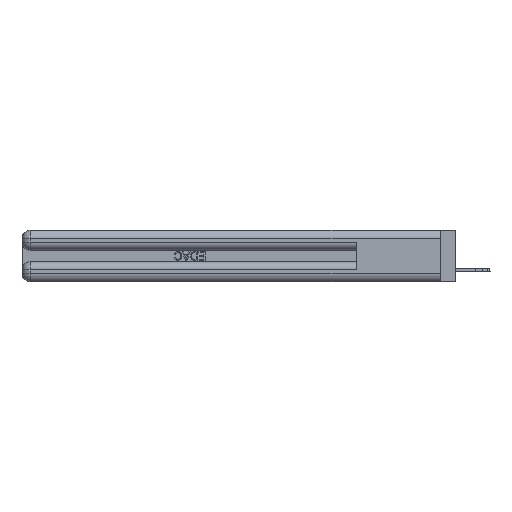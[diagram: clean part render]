
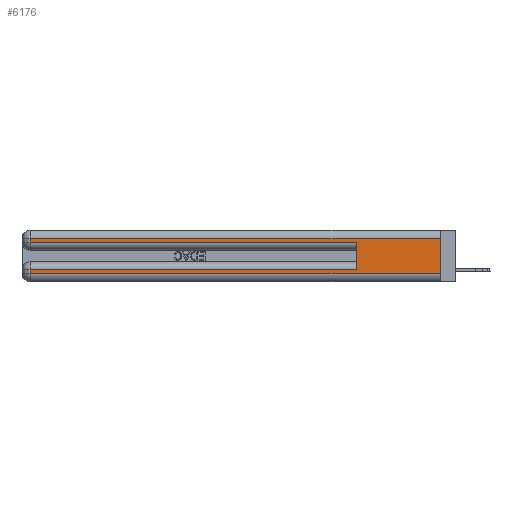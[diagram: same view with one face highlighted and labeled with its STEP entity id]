
A CAD part, left-side view. The second image highlights one B-rep face of the part: STEP entity #6176.
In plain terms, the highlighted planar face has unit normal (-1, 0, 0).
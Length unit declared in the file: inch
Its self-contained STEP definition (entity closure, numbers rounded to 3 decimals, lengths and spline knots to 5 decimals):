
#137 = VECTOR ( 'NONE', #31216, 39.37008 ) ;
#345 = LINE ( 'NONE', #1351, #2214 ) ;
#438 = CARTESIAN_POINT ( 'NONE',  ( 0., 2.94, 0.31 ) ) ;
#1036 = VERTEX_POINT ( 'NONE', #12474 ) ;
#1351 = CARTESIAN_POINT ( 'NONE',  ( 0., 0., 0.06 ) ) ;
#2214 = VECTOR ( 'NONE', #32761, 39.37008 ) ;
#3467 = EDGE_CURVE ( 'NONE', #27188, #27209, #14684, .T. ) ;
#3715 = CARTESIAN_POINT ( 'NONE',  ( 0., 0., 0.085 ) ) ;
#4035 = CARTESIAN_POINT ( 'NONE',  ( 0., 2.94, 0.37 ) ) ;
#4334 = VECTOR ( 'NONE', #23297, 39.37008 ) ;
#4634 = VERTEX_POINT ( 'NONE', #15870 ) ;
#5764 = VECTOR ( 'NONE', #19563, 39.37008 ) ;
#5953 = EDGE_CURVE ( 'NONE', #27188, #14631, #26612, .T. ) ;
#6176 = ADVANCED_FACE ( 'NONE', ( #19824 ), #19379, .F. ) ;
#6967 = CARTESIAN_POINT ( 'NONE',  ( 0., 0., 0.31 ) ) ;
#7120 = VECTOR ( 'NONE', #9620, 39.37008 ) ;
#7391 = ORIENTED_EDGE ( 'NONE', *, *, #26085, .T. ) ;
#7917 = CARTESIAN_POINT ( 'NONE',  ( 0., 0., 0.37 ) ) ;
#8998 = CARTESIAN_POINT ( 'NONE',  ( 0., 0., 0.06 ) ) ;
#9620 = DIRECTION ( 'NONE',  ( 0., 0., -1. ) ) ;
#10275 = LINE ( 'NONE', #4035, #7120 ) ;
#12474 = CARTESIAN_POINT ( 'NONE',  ( 0., 0.6, 0.285 ) ) ;
#12992 = LINE ( 'NONE', #3715, #25179 ) ;
#13042 = EDGE_LOOP ( 'NONE', ( #15852, #16798, #23160, #28432, #29579, #7391, #15346, #23369 ) ) ;
#14120 = AXIS2_PLACEMENT_3D ( 'NONE', #22549, #36945, #28385 ) ;
#14631 = VERTEX_POINT ( 'NONE', #438 ) ;
#14677 = EDGE_CURVE ( 'NONE', #34842, #27209, #345, .T. ) ;
#14684 = LINE ( 'NONE', #7917, #4334 ) ;
#15006 = EDGE_CURVE ( 'NONE', #4634, #1036, #29665, .T. ) ;
#15346 = ORIENTED_EDGE ( 'NONE', *, *, #29931, .T. ) ;
#15852 = ORIENTED_EDGE ( 'NONE', *, *, #3467, .F. ) ;
#15870 = CARTESIAN_POINT ( 'NONE',  ( 0., 2.94, 0.285 ) ) ;
#16798 = ORIENTED_EDGE ( 'NONE', *, *, #5953, .T. ) ;
#17837 = CARTESIAN_POINT ( 'NONE',  ( 0., 2.94, 0.06 ) ) ;
#19379 = PLANE ( 'NONE',  #14120 ) ;
#19454 = EDGE_CURVE ( 'NONE', #14631, #4634, #10275, .T. ) ;
#19563 = DIRECTION ( 'NONE',  ( 0., -1., 0. ) ) ;
#19824 = FACE_OUTER_BOUND ( 'NONE', #13042, .T. ) ;
#21332 = DIRECTION ( 'NONE',  ( 0., 1., 0. ) ) ;
#22549 = CARTESIAN_POINT ( 'NONE',  ( 0., 0., 0.37 ) ) ;
#23160 = ORIENTED_EDGE ( 'NONE', *, *, #19454, .T. ) ;
#23297 = DIRECTION ( 'NONE',  ( 0., 0., -1. ) ) ;
#23369 = ORIENTED_EDGE ( 'NONE', *, *, #14677, .T. ) ;
#25179 = VECTOR ( 'NONE', #21332, 39.37008 ) ;
#25844 = LINE ( 'NONE', #34040, #137 ) ;
#26085 = EDGE_CURVE ( 'NONE', #35546, #35558, #12992, .T. ) ;
#26132 = EDGE_CURVE ( 'NONE', #35546, #1036, #31992, .T. ) ;
#26612 = LINE ( 'NONE', #28768, #27999 ) ;
#27188 = VERTEX_POINT ( 'NONE', #6967 ) ;
#27209 = VERTEX_POINT ( 'NONE', #8998 ) ;
#27428 = VECTOR ( 'NONE', #29947, 39.37008 ) ;
#27999 = VECTOR ( 'NONE', #37109, 39.37008 ) ;
#28385 = DIRECTION ( 'NONE',  ( 0., 0., -1. ) ) ;
#28432 = ORIENTED_EDGE ( 'NONE', *, *, #15006, .T. ) ;
#28768 = CARTESIAN_POINT ( 'NONE',  ( 0., 0., 0.31 ) ) ;
#29426 = CARTESIAN_POINT ( 'NONE',  ( 0., 0.6, 0.085 ) ) ;
#29579 = ORIENTED_EDGE ( 'NONE', *, *, #26132, .F. ) ;
#29665 = LINE ( 'NONE', #36995, #5764 ) ;
#29681 = CARTESIAN_POINT ( 'NONE',  ( 0., 2.94, 0.085 ) ) ;
#29931 = EDGE_CURVE ( 'NONE', #35558, #34842, #25844, .T. ) ;
#29947 = DIRECTION ( 'NONE',  ( 0., 0., 1. ) ) ;
#30084 = CARTESIAN_POINT ( 'NONE',  ( 0., 0.6, 0.145 ) ) ;
#31216 = DIRECTION ( 'NONE',  ( 0., 0., -1. ) ) ;
#31992 = LINE ( 'NONE', #30084, #27428 ) ;
#32761 = DIRECTION ( 'NONE',  ( 0., -1., 0. ) ) ;
#34040 = CARTESIAN_POINT ( 'NONE',  ( 0., 2.94, 0.37 ) ) ;
#34842 = VERTEX_POINT ( 'NONE', #17837 ) ;
#35546 = VERTEX_POINT ( 'NONE', #29426 ) ;
#35558 = VERTEX_POINT ( 'NONE', #29681 ) ;
#36945 = DIRECTION ( 'NONE',  ( 1., 0., 0. ) ) ;
#36995 = CARTESIAN_POINT ( 'NONE',  ( 0., 0., 0.285 ) ) ;
#37109 = DIRECTION ( 'NONE',  ( 0., 1., 0. ) ) ;
